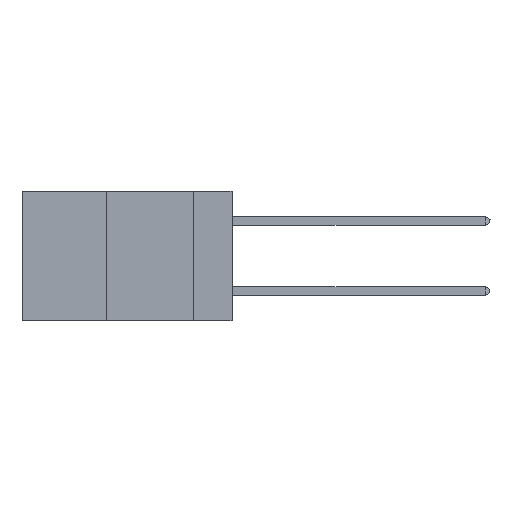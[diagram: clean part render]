
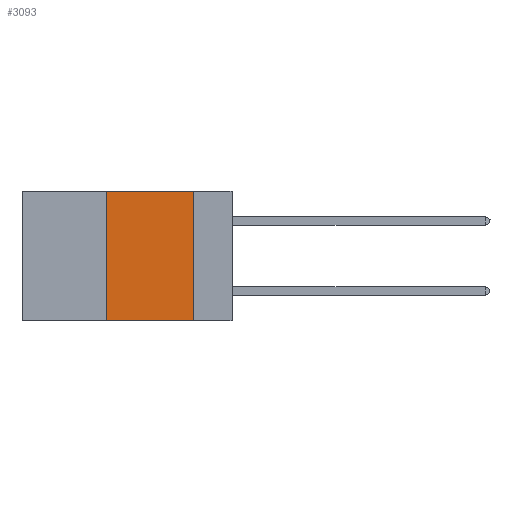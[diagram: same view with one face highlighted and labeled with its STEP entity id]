
A CAD part, left-side view. The second image highlights one B-rep face of the part: STEP entity #3093.
In plain terms, the highlighted planar face has unit normal (-1, 0, 0).
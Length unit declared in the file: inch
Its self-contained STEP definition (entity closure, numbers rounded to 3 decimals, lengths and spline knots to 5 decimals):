
#338 = VERTEX_POINT ( 'NONE', #6592 ) ;
#584 = LINE ( 'NONE', #10839, #5786 ) ;
#1539 = CARTESIAN_POINT ( 'NONE',  ( 0., 0.6, 0. ) ) ;
#2602 = DIRECTION ( 'NONE',  ( 0., 0., 1. ) ) ;
#3093 = ADVANCED_FACE ( 'NONE', ( #3670 ), #8777, .F. ) ;
#3521 = LINE ( 'NONE', #18766, #16719 ) ;
#3670 = FACE_OUTER_BOUND ( 'NONE', #9909, .T. ) ;
#5602 = CARTESIAN_POINT ( 'NONE',  ( 0., 0.36, -0.37 ) ) ;
#5786 = VECTOR ( 'NONE', #9272, 39.37008 ) ;
#6592 = CARTESIAN_POINT ( 'NONE',  ( 0., 0.36, 0. ) ) ;
#8455 = VERTEX_POINT ( 'NONE', #5602 ) ;
#8777 = PLANE ( 'NONE',  #10729 ) ;
#9272 = DIRECTION ( 'NONE',  ( 0., -1., 0. ) ) ;
#9833 = EDGE_CURVE ( 'NONE', #18835, #13977, #15349, .T. ) ;
#9909 = EDGE_LOOP ( 'NONE', ( #11229, #14359, #20398, #18057 ) ) ;
#9954 = LINE ( 'NONE', #16831, #22010 ) ;
#10413 = DIRECTION ( 'NONE',  ( 0., -1., 0. ) ) ;
#10729 = AXIS2_PLACEMENT_3D ( 'NONE', #1539, #15662, #13620 ) ;
#10839 = CARTESIAN_POINT ( 'NONE',  ( 0., 0.6, -0.37 ) ) ;
#11229 = ORIENTED_EDGE ( 'NONE', *, *, #9833, .F. ) ;
#11841 = DIRECTION ( 'NONE',  ( 0., 0., -1. ) ) ;
#13154 = CARTESIAN_POINT ( 'NONE',  ( 0., 0.11, 0. ) ) ;
#13620 = DIRECTION ( 'NONE',  ( 0., 0., -1. ) ) ;
#13878 = CARTESIAN_POINT ( 'NONE',  ( 0., 0.11, 0. ) ) ;
#13977 = VERTEX_POINT ( 'NONE', #21985 ) ;
#14359 = ORIENTED_EDGE ( 'NONE', *, *, #16456, .F. ) ;
#14746 = VECTOR ( 'NONE', #11841, 39.37008 ) ;
#15349 = LINE ( 'NONE', #13878, #14746 ) ;
#15662 = DIRECTION ( 'NONE',  ( 1., 0., 0. ) ) ;
#16456 = EDGE_CURVE ( 'NONE', #338, #18835, #3521, .T. ) ;
#16719 = VECTOR ( 'NONE', #10413, 39.37008 ) ;
#16831 = CARTESIAN_POINT ( 'NONE',  ( 0., 0.36, 0. ) ) ;
#18057 = ORIENTED_EDGE ( 'NONE', *, *, #19169, .T. ) ;
#18766 = CARTESIAN_POINT ( 'NONE',  ( 0., 0.6, 0. ) ) ;
#18835 = VERTEX_POINT ( 'NONE', #13154 ) ;
#19169 = EDGE_CURVE ( 'NONE', #8455, #13977, #584, .T. ) ;
#19370 = EDGE_CURVE ( 'NONE', #8455, #338, #9954, .T. ) ;
#20398 = ORIENTED_EDGE ( 'NONE', *, *, #19370, .F. ) ;
#21985 = CARTESIAN_POINT ( 'NONE',  ( 0., 0.11, -0.37 ) ) ;
#22010 = VECTOR ( 'NONE', #2602, 39.37008 ) ;
